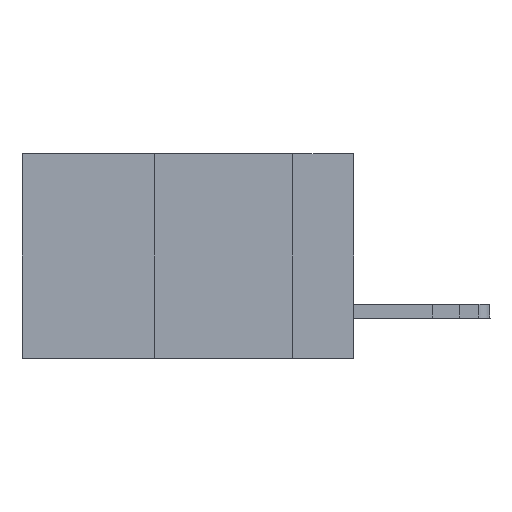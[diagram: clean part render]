
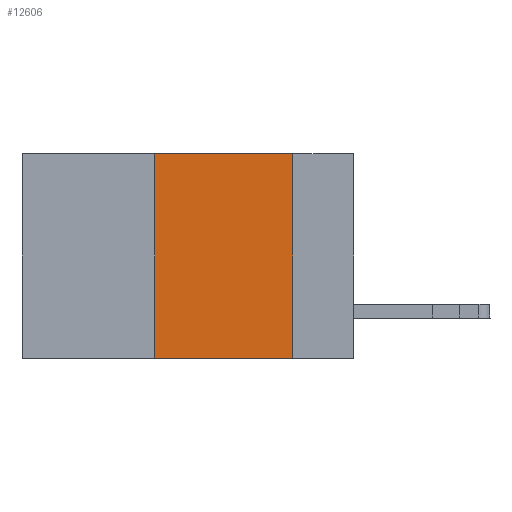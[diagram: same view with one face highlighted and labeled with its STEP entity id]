
A CAD part, left-side view. The second image highlights one B-rep face of the part: STEP entity #12606.
In plain terms, the highlighted planar face has unit normal (-1, 0, 0).
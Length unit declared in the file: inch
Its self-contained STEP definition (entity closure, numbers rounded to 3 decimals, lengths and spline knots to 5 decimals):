
#133 = DIRECTION ( 'NONE',  ( 0., 0., -1. ) ) ;
#377 = EDGE_CURVE ( 'NONE', #9619, #20911, #16736, .T. ) ;
#1745 = LINE ( 'NONE', #15457, #19627 ) ;
#3555 = VERTEX_POINT ( 'NONE', #4988 ) ;
#4293 = CARTESIAN_POINT ( 'NONE',  ( 0., 0.36, 0. ) ) ;
#4396 = CARTESIAN_POINT ( 'NONE',  ( 0., 0.36, -0.37 ) ) ;
#4495 = LINE ( 'NONE', #20869, #16677 ) ;
#4988 = CARTESIAN_POINT ( 'NONE',  ( 0., 0.11, -0.37 ) ) ;
#6560 = CARTESIAN_POINT ( 'NONE',  ( 0., 0.6, 0. ) ) ;
#7246 = DIRECTION ( 'NONE',  ( 0., -1., 0. ) ) ;
#7299 = EDGE_CURVE ( 'NONE', #9619, #3555, #4495, .T. ) ;
#7573 = DIRECTION ( 'NONE',  ( 0., 0., 1. ) ) ;
#8327 = VERTEX_POINT ( 'NONE', #14133 ) ;
#8388 = DIRECTION ( 'NONE',  ( 1., 0., 0. ) ) ;
#8582 = LINE ( 'NONE', #13082, #17499 ) ;
#8970 = CARTESIAN_POINT ( 'NONE',  ( 0., 0.36, 0. ) ) ;
#9619 = VERTEX_POINT ( 'NONE', #4396 ) ;
#9692 = ORIENTED_EDGE ( 'NONE', *, *, #14554, .F. ) ;
#11748 = ORIENTED_EDGE ( 'NONE', *, *, #7299, .T. ) ;
#12396 = EDGE_LOOP ( 'NONE', ( #14802, #9692, #19164, #11748 ) ) ;
#12425 = VECTOR ( 'NONE', #7573, 39.37008 ) ;
#12606 = ADVANCED_FACE ( 'NONE', ( #13040 ), #17847, .F. ) ;
#12929 = AXIS2_PLACEMENT_3D ( 'NONE', #6560, #8388, #19770 ) ;
#13040 = FACE_OUTER_BOUND ( 'NONE', #12396, .T. ) ;
#13082 = CARTESIAN_POINT ( 'NONE',  ( 0., 0.11, 0. ) ) ;
#14133 = CARTESIAN_POINT ( 'NONE',  ( 0., 0.11, 0. ) ) ;
#14554 = EDGE_CURVE ( 'NONE', #20911, #8327, #1745, .T. ) ;
#14802 = ORIENTED_EDGE ( 'NONE', *, *, #16623, .F. ) ;
#15457 = CARTESIAN_POINT ( 'NONE',  ( 0., 0.6, 0. ) ) ;
#16623 = EDGE_CURVE ( 'NONE', #8327, #3555, #8582, .T. ) ;
#16677 = VECTOR ( 'NONE', #18696, 39.37008 ) ;
#16736 = LINE ( 'NONE', #4293, #12425 ) ;
#17499 = VECTOR ( 'NONE', #133, 39.37008 ) ;
#17847 = PLANE ( 'NONE',  #12929 ) ;
#18696 = DIRECTION ( 'NONE',  ( 0., -1., 0. ) ) ;
#19164 = ORIENTED_EDGE ( 'NONE', *, *, #377, .F. ) ;
#19627 = VECTOR ( 'NONE', #7246, 39.37008 ) ;
#19770 = DIRECTION ( 'NONE',  ( 0., 0., -1. ) ) ;
#20869 = CARTESIAN_POINT ( 'NONE',  ( 0., 0.6, -0.37 ) ) ;
#20911 = VERTEX_POINT ( 'NONE', #8970 ) ;
